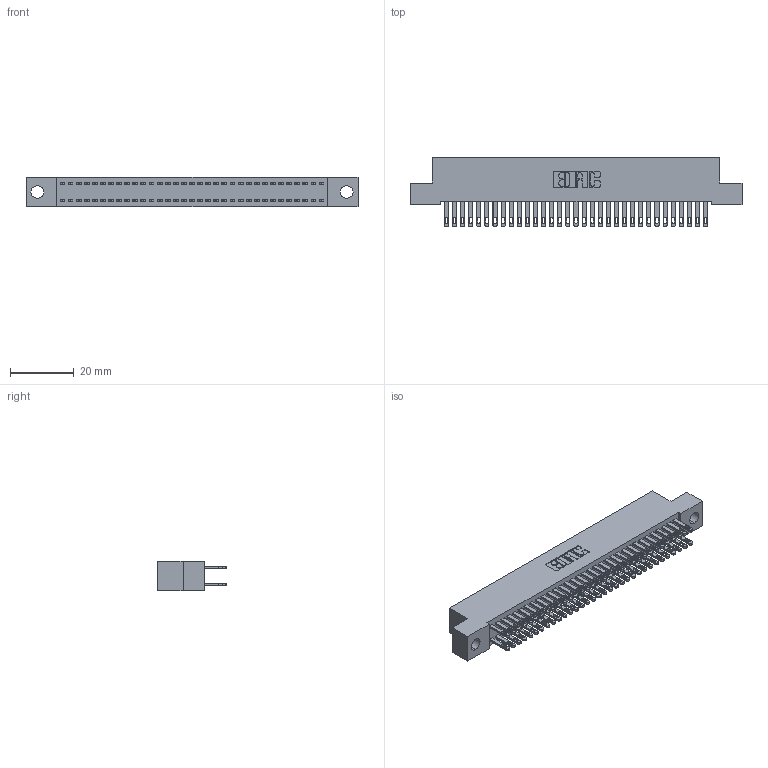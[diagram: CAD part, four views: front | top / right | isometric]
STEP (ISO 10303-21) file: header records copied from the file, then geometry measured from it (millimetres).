
FILE_DESCRIPTION (( 'STEP AP203' ), '1' );
FILE_NAME ('342-066-500-204.STEP', '2018-08-13T07:46:28', ( '' ), ( '' ), 'SwSTEP 2.0', 'SolidWorks 2016', '' );
FILE_SCHEMA (( 'CONFIG_CONTROL_DESIGN' ));
Length unit declared in the file: inch
Products named in the file (3): 345-292-001_345-293-100; 342-066-500-204; 342 Part_.156 TH
Assembly tree (67 placements, depth 2):
  342-066-500-204
    342 Part_.156 TH
    345-292-001_345-293-100  x66
Bounding box: 104.14 x 21.85 x 9.4 mm (x, y, z)
Volume: 9429 mm3; surface area: 15582.4 mm2
Topology: 67 solids, 67 shells, 3278 faces, 10001 edges, 6666 vertices
Faces by surface type: plane 2046, cylinder 1232
Entity records: 22195 total; most frequent: CARTESIAN_POINT 3686, ORIENTED_EDGE 3622, DIRECTION 3167, EDGE_CURVE 1811, LINE 1679, VECTOR 1679, VERTEX_POINT 1206, AXIS2_PLACEMENT_3D 744
